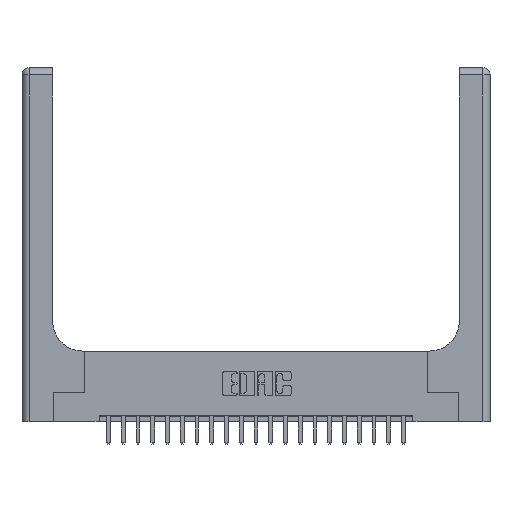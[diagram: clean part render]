
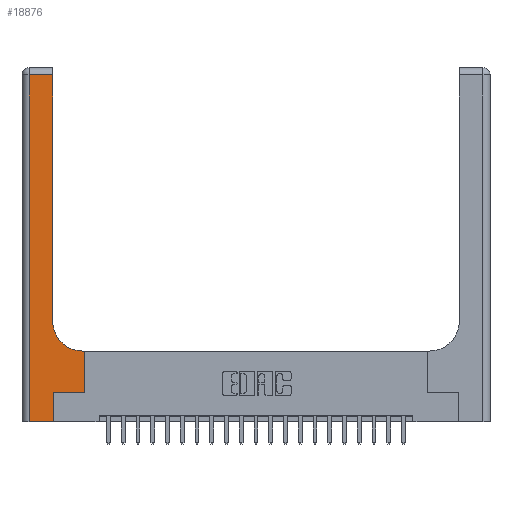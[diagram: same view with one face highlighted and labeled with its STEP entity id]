
A CAD part, top view. The second image highlights one B-rep face of the part: STEP entity #18876.
In plain terms, the highlighted planar face has unit normal (0, 0, 1).
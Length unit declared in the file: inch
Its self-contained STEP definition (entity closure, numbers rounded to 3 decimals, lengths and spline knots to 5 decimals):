
#407 = CARTESIAN_POINT ( 'NONE',  ( 0.528, 0.25, 0.37 ) ) ;
#624 = VECTOR ( 'NONE', #16225, 39.37008 ) ;
#1052 = VERTEX_POINT ( 'NONE', #1662 ) ;
#1143 = VECTOR ( 'NONE', #4830, 39.37008 ) ;
#1662 = CARTESIAN_POINT ( 'NONE',  ( 0.265, 0.25, 0.37 ) ) ;
#2238 = LINE ( 'NONE', #5320, #2503 ) ;
#2314 = CARTESIAN_POINT ( 'NONE',  ( 0., 2.94, 0.37 ) ) ;
#2503 = VECTOR ( 'NONE', #10388, 39.37008 ) ;
#2575 = ORIENTED_EDGE ( 'NONE', *, *, #16182, .T. ) ;
#2775 = EDGE_CURVE ( 'NONE', #1052, #21130, #10841, .T. ) ;
#3013 = VERTEX_POINT ( 'NONE', #19178 ) ;
#3199 = VERTEX_POINT ( 'NONE', #19529 ) ;
#3319 = CARTESIAN_POINT ( 'NONE',  ( 0.265, 0.25, 0.37 ) ) ;
#3579 = VERTEX_POINT ( 'NONE', #7357 ) ;
#3839 = VECTOR ( 'NONE', #13559, 39.37008 ) ;
#3909 = EDGE_CURVE ( 'NONE', #21130, #3199, #10131, .T. ) ;
#4005 = ORIENTED_EDGE ( 'NONE', *, *, #11064, .T. ) ;
#4019 = CARTESIAN_POINT ( 'NONE',  ( 0.51, 0.6, 0.37 ) ) ;
#4830 = DIRECTION ( 'NONE',  ( -1., 0., 0. ) ) ;
#5045 = DIRECTION ( 'NONE',  ( 1., 0., 0. ) ) ;
#5320 = CARTESIAN_POINT ( 'NONE',  ( 0.06, 3., 0.37 ) ) ;
#5665 = LINE ( 'NONE', #16387, #1143 ) ;
#5927 = EDGE_CURVE ( 'NONE', #17674, #8730, #8225, .T. ) ;
#7357 = CARTESIAN_POINT ( 'NONE',  ( 0.06, 0., 0.37 ) ) ;
#7833 = VERTEX_POINT ( 'NONE', #16237 ) ;
#7879 = DIRECTION ( 'NONE',  ( -1., 0., 0. ) ) ;
#8225 = CIRCLE ( 'NONE', #14332, 0.25 ) ;
#8308 = LINE ( 'NONE', #15794, #10934 ) ;
#8418 = FACE_OUTER_BOUND ( 'NONE', #15460, .T. ) ;
#8586 = CARTESIAN_POINT ( 'NONE',  ( 0.528, 0.25, 0.37 ) ) ;
#8691 = ORIENTED_EDGE ( 'NONE', *, *, #3909, .T. ) ;
#8730 = VERTEX_POINT ( 'NONE', #11758 ) ;
#8879 = EDGE_CURVE ( 'NONE', #14210, #3579, #2238, .T. ) ;
#9062 = VECTOR ( 'NONE', #13439, 39.37008 ) ;
#9627 = CARTESIAN_POINT ( 'NONE',  ( 0.51, 0.85, 0.37 ) ) ;
#9701 = PLANE ( 'NONE',  #13088 ) ;
#9772 = ORIENTED_EDGE ( 'NONE', *, *, #5927, .T. ) ;
#9870 = EDGE_CURVE ( 'NONE', #3579, #7833, #8308, .T. ) ;
#9946 = EDGE_CURVE ( 'NONE', #8730, #3013, #18288, .T. ) ;
#10131 = LINE ( 'NONE', #8586, #9062 ) ;
#10388 = DIRECTION ( 'NONE',  ( 0., -1., 0. ) ) ;
#10841 = LINE ( 'NONE', #3319, #19825 ) ;
#10934 = VECTOR ( 'NONE', #19216, 39.37008 ) ;
#11064 = EDGE_CURVE ( 'NONE', #3013, #14210, #18799, .T. ) ;
#11122 = CARTESIAN_POINT ( 'NONE',  ( 0.06, 2.94, 0.37 ) ) ;
#11758 = CARTESIAN_POINT ( 'NONE',  ( 0.26, 0.85, 0.37 ) ) ;
#12779 = CARTESIAN_POINT ( 'NONE',  ( 0.26, 3., 0.37 ) ) ;
#13088 = AXIS2_PLACEMENT_3D ( 'NONE', #14567, #21346, #7879 ) ;
#13439 = DIRECTION ( 'NONE',  ( 0., 1., 0. ) ) ;
#13559 = DIRECTION ( 'NONE',  ( 0., 1., 0. ) ) ;
#13738 = ORIENTED_EDGE ( 'NONE', *, *, #9946, .T. ) ;
#14185 = ORIENTED_EDGE ( 'NONE', *, *, #20991, .T. ) ;
#14210 = VERTEX_POINT ( 'NONE', #11122 ) ;
#14332 = AXIS2_PLACEMENT_3D ( 'NONE', #9627, #20009, #21413 ) ;
#14567 = CARTESIAN_POINT ( 'NONE',  ( 0., 3., 0.37 ) ) ;
#15309 = CARTESIAN_POINT ( 'NONE',  ( 0.265, 0., 0.37 ) ) ;
#15460 = EDGE_LOOP ( 'NONE', ( #13738, #4005, #19272, #19533, #14185, #15538, #8691, #2575, #9772 ) ) ;
#15538 = ORIENTED_EDGE ( 'NONE', *, *, #2775, .T. ) ;
#15794 = CARTESIAN_POINT ( 'NONE',  ( 0., 0., 0.37 ) ) ;
#16182 = EDGE_CURVE ( 'NONE', #3199, #17674, #5665, .T. ) ;
#16225 = DIRECTION ( 'NONE',  ( 0., 1., 0. ) ) ;
#16237 = CARTESIAN_POINT ( 'NONE',  ( 0.265, 0., 0.37 ) ) ;
#16387 = CARTESIAN_POINT ( 'NONE',  ( 0.26, 0.6, 0.37 ) ) ;
#17674 = VERTEX_POINT ( 'NONE', #4019 ) ;
#18288 = LINE ( 'NONE', #12779, #624 ) ;
#18799 = LINE ( 'NONE', #2314, #19855 ) ;
#18876 = ADVANCED_FACE ( 'NONE', ( #8418 ), #9701, .F. ) ;
#18932 = DIRECTION ( 'NONE',  ( -1., 0., 0. ) ) ;
#19178 = CARTESIAN_POINT ( 'NONE',  ( 0.26, 2.94, 0.37 ) ) ;
#19216 = DIRECTION ( 'NONE',  ( 1., 0., 0. ) ) ;
#19272 = ORIENTED_EDGE ( 'NONE', *, *, #8879, .T. ) ;
#19529 = CARTESIAN_POINT ( 'NONE',  ( 0.528, 0.6, 0.37 ) ) ;
#19533 = ORIENTED_EDGE ( 'NONE', *, *, #9870, .T. ) ;
#19825 = VECTOR ( 'NONE', #5045, 39.37008 ) ;
#19855 = VECTOR ( 'NONE', #18932, 39.37008 ) ;
#20009 = DIRECTION ( 'NONE',  ( 0., 0., -1. ) ) ;
#20991 = EDGE_CURVE ( 'NONE', #7833, #1052, #21516, .T. ) ;
#21130 = VERTEX_POINT ( 'NONE', #407 ) ;
#21346 = DIRECTION ( 'NONE',  ( 0., 0., -1. ) ) ;
#21413 = DIRECTION ( 'NONE',  ( 1., 0., 0. ) ) ;
#21516 = LINE ( 'NONE', #15309, #3839 ) ;
